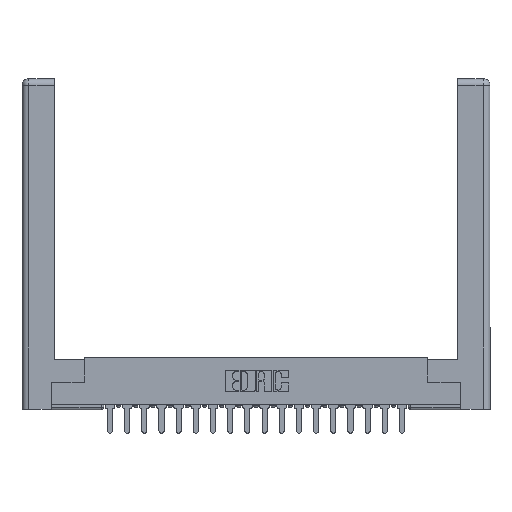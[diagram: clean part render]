
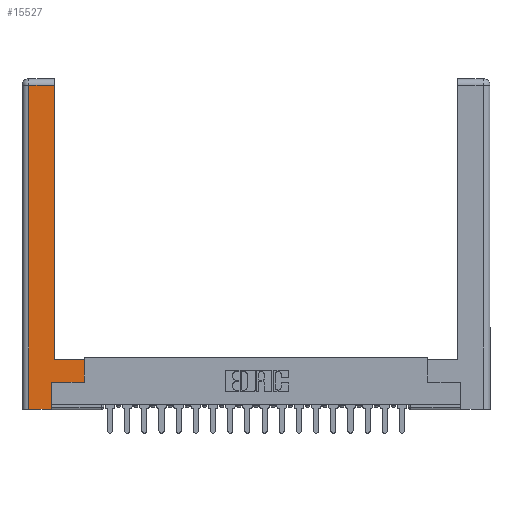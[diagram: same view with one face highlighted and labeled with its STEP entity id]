
A CAD part, top view. The second image highlights one B-rep face of the part: STEP entity #15527.
In plain terms, the highlighted planar face has unit normal (0, 0, 1).
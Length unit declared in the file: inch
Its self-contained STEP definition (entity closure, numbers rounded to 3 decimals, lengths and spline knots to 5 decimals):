
#71 = VECTOR ( 'NONE', #619, 39.37008 ) ;
#390 = VECTOR ( 'NONE', #13196, 39.37008 ) ;
#581 = EDGE_CURVE ( 'NONE', #17520, #8841, #8989, .T. ) ;
#619 = DIRECTION ( 'NONE',  ( 0., 1., 0. ) ) ;
#713 = EDGE_CURVE ( 'NONE', #16819, #19185, #17626, .T. ) ;
#743 = ORIENTED_EDGE ( 'NONE', *, *, #2934, .T. ) ;
#1011 = CARTESIAN_POINT ( 'NONE',  ( 0.565, 0.45, 0. ) ) ;
#1372 = DIRECTION ( 'NONE',  ( -1., 0., 0. ) ) ;
#1412 = CARTESIAN_POINT ( 'NONE',  ( 0.0615, 2.94, 0. ) ) ;
#1700 = DIRECTION ( 'NONE',  ( 1., 0., 0. ) ) ;
#1980 = VECTOR ( 'NONE', #7817, 39.37008 ) ;
#2240 = VERTEX_POINT ( 'NONE', #1011 ) ;
#2912 = LINE ( 'NONE', #8331, #19129 ) ;
#2934 = EDGE_CURVE ( 'NONE', #3319, #2240, #2912, .T. ) ;
#3128 = CARTESIAN_POINT ( 'NONE',  ( 0.0615, 0., 0. ) ) ;
#3133 = EDGE_CURVE ( 'NONE', #13648, #12067, #13360, .T. ) ;
#3241 = VECTOR ( 'NONE', #18252, 39.37008 ) ;
#3319 = VERTEX_POINT ( 'NONE', #7806 ) ;
#3740 = CARTESIAN_POINT ( 'NONE',  ( 0.265, 0.245, 0. ) ) ;
#4114 = EDGE_CURVE ( 'NONE', #12067, #3319, #14082, .T. ) ;
#4538 = DIRECTION ( 'NONE',  ( -1., 0., 0. ) ) ;
#5119 = CARTESIAN_POINT ( 'NONE',  ( 0.265, 0., 0. ) ) ;
#5325 = CARTESIAN_POINT ( 'NONE',  ( 0.295, 2.94, 0. ) ) ;
#5979 = VECTOR ( 'NONE', #8791, 39.37008 ) ;
#6734 = DIRECTION ( 'NONE',  ( 0., 1., 0. ) ) ;
#6942 = LINE ( 'NONE', #16145, #1980 ) ;
#7516 = ORIENTED_EDGE ( 'NONE', *, *, #3133, .T. ) ;
#7586 = LINE ( 'NONE', #5119, #12542 ) ;
#7705 = EDGE_LOOP ( 'NONE', ( #12157, #15411, #10384, #9491, #7516, #17474, #743, #10868 ) ) ;
#7806 = CARTESIAN_POINT ( 'NONE',  ( 0.565, 0.245, 0. ) ) ;
#7817 = DIRECTION ( 'NONE',  ( -1., 0., 0. ) ) ;
#8331 = CARTESIAN_POINT ( 'NONE',  ( 0.565, 0.45, 0. ) ) ;
#8791 = DIRECTION ( 'NONE',  ( 1., 0., 0. ) ) ;
#8841 = VERTEX_POINT ( 'NONE', #5325 ) ;
#8989 = LINE ( 'NONE', #18031, #390 ) ;
#9491 = ORIENTED_EDGE ( 'NONE', *, *, #11804, .T. ) ;
#10164 = FACE_OUTER_BOUND ( 'NONE', #7705, .T. ) ;
#10384 = ORIENTED_EDGE ( 'NONE', *, *, #713, .T. ) ;
#10868 = ORIENTED_EDGE ( 'NONE', *, *, #18638, .T. ) ;
#11719 = CARTESIAN_POINT ( 'NONE',  ( 0.295, 0.45, 0. ) ) ;
#11804 = EDGE_CURVE ( 'NONE', #19185, #13648, #7586, .T. ) ;
#12067 = VERTEX_POINT ( 'NONE', #12194 ) ;
#12157 = ORIENTED_EDGE ( 'NONE', *, *, #581, .T. ) ;
#12194 = CARTESIAN_POINT ( 'NONE',  ( 0.265, 0.245, 0. ) ) ;
#12542 = VECTOR ( 'NONE', #1700, 39.37008 ) ;
#13196 = DIRECTION ( 'NONE',  ( 0., 1., 0. ) ) ;
#13360 = LINE ( 'NONE', #3740, #71 ) ;
#13648 = VERTEX_POINT ( 'NONE', #18084 ) ;
#14082 = LINE ( 'NONE', #18744, #5979 ) ;
#14542 = CARTESIAN_POINT ( 'NONE',  ( 0.0615, 2.94, 0. ) ) ;
#14871 = VECTOR ( 'NONE', #4538, 39.37008 ) ;
#15411 = ORIENTED_EDGE ( 'NONE', *, *, #20877, .T. ) ;
#15527 = ADVANCED_FACE ( 'NONE', ( #10164 ), #19853, .F. ) ;
#16145 = CARTESIAN_POINT ( 'NONE',  ( 0.295, 0.45, 0. ) ) ;
#16819 = VERTEX_POINT ( 'NONE', #1412 ) ;
#17474 = ORIENTED_EDGE ( 'NONE', *, *, #4114, .T. ) ;
#17520 = VERTEX_POINT ( 'NONE', #11719 ) ;
#17626 = LINE ( 'NONE', #3128, #3241 ) ;
#18031 = CARTESIAN_POINT ( 'NONE',  ( 0.295, 3., 0. ) ) ;
#18084 = CARTESIAN_POINT ( 'NONE',  ( 0.265, 0., 0. ) ) ;
#18252 = DIRECTION ( 'NONE',  ( 0., -1., 0. ) ) ;
#18638 = EDGE_CURVE ( 'NONE', #2240, #17520, #6942, .T. ) ;
#18744 = CARTESIAN_POINT ( 'NONE',  ( 0.565, 0.245, 0. ) ) ;
#19129 = VECTOR ( 'NONE', #6734, 39.37008 ) ;
#19185 = VERTEX_POINT ( 'NONE', #19891 ) ;
#19708 = DIRECTION ( 'NONE',  ( 0., 0., -1. ) ) ;
#19853 = PLANE ( 'NONE',  #20410 ) ;
#19891 = CARTESIAN_POINT ( 'NONE',  ( 0.0615, 0., 0. ) ) ;
#20377 = LINE ( 'NONE', #14542, #14871 ) ;
#20410 = AXIS2_PLACEMENT_3D ( 'NONE', #21300, #19708, #1372 ) ;
#20877 = EDGE_CURVE ( 'NONE', #8841, #16819, #20377, .T. ) ;
#21300 = CARTESIAN_POINT ( 'NONE',  ( 0., 0., 0. ) ) ;
